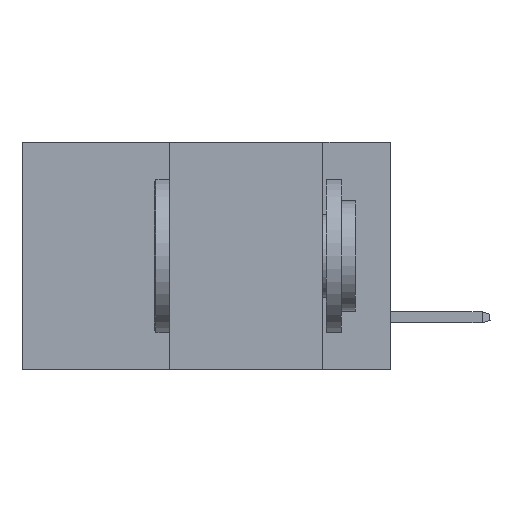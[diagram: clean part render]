
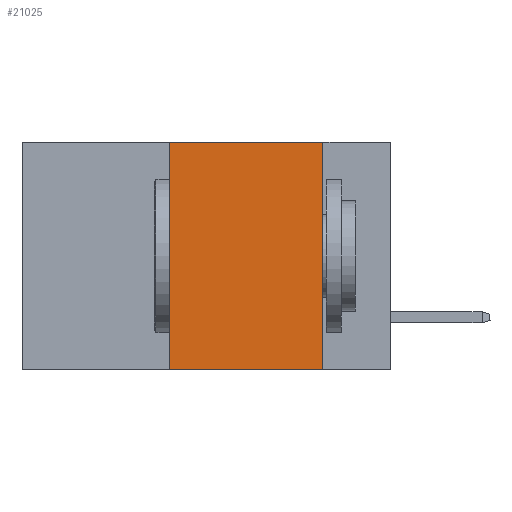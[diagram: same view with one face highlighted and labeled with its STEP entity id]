
A CAD part, left-side view. The second image highlights one B-rep face of the part: STEP entity #21025.
In plain terms, the highlighted planar face has unit normal (-1, 0, 0).
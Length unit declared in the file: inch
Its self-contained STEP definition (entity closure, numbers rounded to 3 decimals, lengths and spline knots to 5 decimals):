
#553 = CARTESIAN_POINT ( 'NONE',  ( 0., 0.36, 0. ) ) ;
#2872 = CARTESIAN_POINT ( 'NONE',  ( 0., 0.6, 0. ) ) ;
#5612 = CARTESIAN_POINT ( 'NONE',  ( 0., 0.36, -0.37 ) ) ;
#8009 = CARTESIAN_POINT ( 'NONE',  ( 0., 0.6, -0.37 ) ) ;
#9981 = VERTEX_POINT ( 'NONE', #44041 ) ;
#10631 = VECTOR ( 'NONE', #37033, 39.37008 ) ;
#12107 = VECTOR ( 'NONE', #22348, 39.37008 ) ;
#14252 = VERTEX_POINT ( 'NONE', #5612 ) ;
#14279 = EDGE_CURVE ( 'NONE', #36540, #39438, #14551, .T. ) ;
#14551 = LINE ( 'NONE', #40677, #19018 ) ;
#16352 = CARTESIAN_POINT ( 'NONE',  ( 0., 0.11, 0. ) ) ;
#16628 = CARTESIAN_POINT ( 'NONE',  ( 0., 0.36, 0. ) ) ;
#18555 = EDGE_CURVE ( 'NONE', #14252, #36540, #20078, .T. ) ;
#19018 = VECTOR ( 'NONE', #44311, 39.37008 ) ;
#20078 = LINE ( 'NONE', #16628, #10631 ) ;
#20901 = EDGE_CURVE ( 'NONE', #14252, #9981, #38002, .T. ) ;
#21025 = ADVANCED_FACE ( 'NONE', ( #35203 ), #33874, .F. ) ;
#22348 = DIRECTION ( 'NONE',  ( 0., -1., 0. ) ) ;
#24072 = ORIENTED_EDGE ( 'NONE', *, *, #42095, .F. ) ;
#26938 = DIRECTION ( 'NONE',  ( 0., 0., -1. ) ) ;
#29003 = ORIENTED_EDGE ( 'NONE', *, *, #18555, .F. ) ;
#30845 = ORIENTED_EDGE ( 'NONE', *, *, #14279, .F. ) ;
#30990 = DIRECTION ( 'NONE',  ( 0., 0., -1. ) ) ;
#33874 = PLANE ( 'NONE',  #34810 ) ;
#34139 = VECTOR ( 'NONE', #26938, 39.37008 ) ;
#34476 = DIRECTION ( 'NONE',  ( 1., 0., 0. ) ) ;
#34810 = AXIS2_PLACEMENT_3D ( 'NONE', #2872, #34476, #30990 ) ;
#35203 = FACE_OUTER_BOUND ( 'NONE', #39594, .T. ) ;
#36540 = VERTEX_POINT ( 'NONE', #553 ) ;
#37033 = DIRECTION ( 'NONE',  ( 0., 0., 1. ) ) ;
#38002 = LINE ( 'NONE', #8009, #12107 ) ;
#38739 = ORIENTED_EDGE ( 'NONE', *, *, #20901, .T. ) ;
#39050 = LINE ( 'NONE', #16352, #34139 ) ;
#39438 = VERTEX_POINT ( 'NONE', #43638 ) ;
#39594 = EDGE_LOOP ( 'NONE', ( #24072, #30845, #29003, #38739 ) ) ;
#40677 = CARTESIAN_POINT ( 'NONE',  ( 0., 0.6, 0. ) ) ;
#42095 = EDGE_CURVE ( 'NONE', #39438, #9981, #39050, .T. ) ;
#43638 = CARTESIAN_POINT ( 'NONE',  ( 0., 0.11, 0. ) ) ;
#44041 = CARTESIAN_POINT ( 'NONE',  ( 0., 0.11, -0.37 ) ) ;
#44311 = DIRECTION ( 'NONE',  ( 0., -1., 0. ) ) ;
